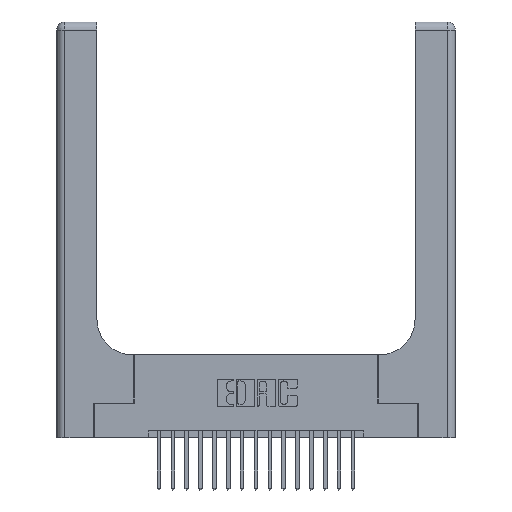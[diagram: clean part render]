
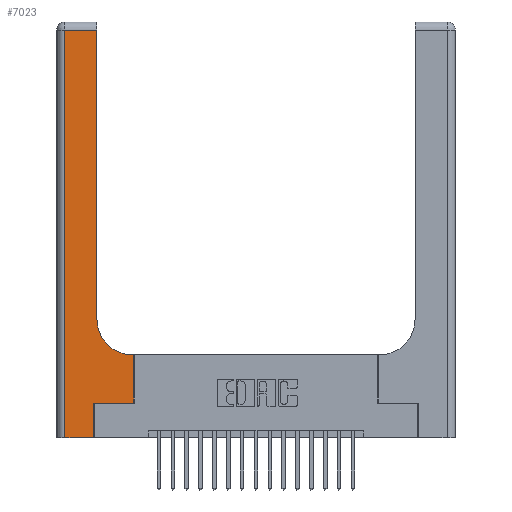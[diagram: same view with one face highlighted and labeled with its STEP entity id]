
A CAD part, top view. The second image highlights one B-rep face of the part: STEP entity #7023.
In plain terms, the highlighted planar face has unit normal (0, 0, 1).
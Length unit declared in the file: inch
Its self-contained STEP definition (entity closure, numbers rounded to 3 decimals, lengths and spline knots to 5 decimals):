
#23 = LINE ( 'NONE', #2422, #16067 ) ;
#148 = VECTOR ( 'NONE', #1297, 39.37008 ) ;
#479 = LINE ( 'NONE', #8664, #4273 ) ;
#485 = DIRECTION ( 'NONE',  ( 1., 0., 0. ) ) ;
#1064 = CARTESIAN_POINT ( 'NONE',  ( 0.06, 2.94, 0.37 ) ) ;
#1297 = DIRECTION ( 'NONE',  ( -1., 0., 0. ) ) ;
#1401 = CARTESIAN_POINT ( 'NONE',  ( 0.2915, 3., 0.37 ) ) ;
#1628 = VERTEX_POINT ( 'NONE', #19528 ) ;
#1999 = LINE ( 'NONE', #17982, #5778 ) ;
#2118 = ORIENTED_EDGE ( 'NONE', *, *, #14097, .T. ) ;
#2130 = CARTESIAN_POINT ( 'NONE',  ( 0.06, 0., 0.37 ) ) ;
#2395 = CARTESIAN_POINT ( 'NONE',  ( 0.5585, 0.25, 0.37 ) ) ;
#2422 = CARTESIAN_POINT ( 'NONE',  ( 0.5585, 0.25, 0.37 ) ) ;
#2802 = ORIENTED_EDGE ( 'NONE', *, *, #19933, .T. ) ;
#3345 = CARTESIAN_POINT ( 'NONE',  ( 0.2915, 0.85, 0.37 ) ) ;
#3592 = EDGE_CURVE ( 'NONE', #9612, #16155, #479, .T. ) ;
#3935 = AXIS2_PLACEMENT_3D ( 'NONE', #5026, #14536, #17753 ) ;
#4273 = VECTOR ( 'NONE', #9222, 39.37008 ) ;
#4458 = LINE ( 'NONE', #6158, #148 ) ;
#5026 = CARTESIAN_POINT ( 'NONE',  ( 0., 3., 0.37 ) ) ;
#5108 = VECTOR ( 'NONE', #8310, 39.37008 ) ;
#5778 = VECTOR ( 'NONE', #6880, 39.37008 ) ;
#5889 = FACE_OUTER_BOUND ( 'NONE', #16660, .T. ) ;
#6094 = LINE ( 'NONE', #17221, #9833 ) ;
#6096 = DIRECTION ( 'NONE',  ( 0., -1., 0. ) ) ;
#6158 = CARTESIAN_POINT ( 'NONE',  ( 0., 2.94, 0.37 ) ) ;
#6204 = CIRCLE ( 'NONE', #20380, 0.25 ) ;
#6464 = VECTOR ( 'NONE', #20124, 39.37008 ) ;
#6644 = PLANE ( 'NONE',  #3935 ) ;
#6880 = DIRECTION ( 'NONE',  ( 0., 1., 0. ) ) ;
#6988 = CARTESIAN_POINT ( 'NONE',  ( 0.269, 0.25, 0.37 ) ) ;
#7023 = ADVANCED_FACE ( 'NONE', ( #5889 ), #6644, .F. ) ;
#7247 = DIRECTION ( 'NONE',  ( 0., 1., 0. ) ) ;
#7655 = CARTESIAN_POINT ( 'NONE',  ( 0.2915, 2.94, 0.37 ) ) ;
#7853 = LINE ( 'NONE', #16240, #5108 ) ;
#8182 = ORIENTED_EDGE ( 'NONE', *, *, #12435, .T. ) ;
#8310 = DIRECTION ( 'NONE',  ( -1., 0., 0. ) ) ;
#8577 = EDGE_CURVE ( 'NONE', #10728, #14247, #18611, .T. ) ;
#8664 = CARTESIAN_POINT ( 'NONE',  ( 0., 0., 0.37 ) ) ;
#8688 = EDGE_CURVE ( 'NONE', #11647, #9305, #4458, .T. ) ;
#9002 = ORIENTED_EDGE ( 'NONE', *, *, #8577, .T. ) ;
#9222 = DIRECTION ( 'NONE',  ( 1., 0., 0. ) ) ;
#9305 = VERTEX_POINT ( 'NONE', #1064 ) ;
#9573 = ORIENTED_EDGE ( 'NONE', *, *, #8688, .T. ) ;
#9612 = VERTEX_POINT ( 'NONE', #2130 ) ;
#9833 = VECTOR ( 'NONE', #6096, 39.37008 ) ;
#10093 = DIRECTION ( 'NONE',  ( 0., 0., -1. ) ) ;
#10425 = ORIENTED_EDGE ( 'NONE', *, *, #17731, .T. ) ;
#10728 = VERTEX_POINT ( 'NONE', #6988 ) ;
#10908 = CARTESIAN_POINT ( 'NONE',  ( 0.5585, 0.6, 0.37 ) ) ;
#10935 = VECTOR ( 'NONE', #14224, 39.37008 ) ;
#10971 = ORIENTED_EDGE ( 'NONE', *, *, #19688, .T. ) ;
#11647 = VERTEX_POINT ( 'NONE', #7655 ) ;
#12234 = ORIENTED_EDGE ( 'NONE', *, *, #3592, .T. ) ;
#12435 = EDGE_CURVE ( 'NONE', #9305, #9612, #6094, .T. ) ;
#14097 = EDGE_CURVE ( 'NONE', #16155, #10728, #1999, .T. ) ;
#14224 = DIRECTION ( 'NONE',  ( 0., 1., 0. ) ) ;
#14247 = VERTEX_POINT ( 'NONE', #2395 ) ;
#14536 = DIRECTION ( 'NONE',  ( 0., 0., -1. ) ) ;
#16067 = VECTOR ( 'NONE', #7247, 39.37008 ) ;
#16155 = VERTEX_POINT ( 'NONE', #20291 ) ;
#16240 = CARTESIAN_POINT ( 'NONE',  ( 0.2915, 0.6, 0.37 ) ) ;
#16660 = EDGE_LOOP ( 'NONE', ( #10425, #9573, #8182, #12234, #2118, #9002, #2802, #10971, #18459 ) ) ;
#16672 = VERTEX_POINT ( 'NONE', #10908 ) ;
#17221 = CARTESIAN_POINT ( 'NONE',  ( 0.06, 3., 0.37 ) ) ;
#17326 = EDGE_CURVE ( 'NONE', #1628, #19629, #6204, .T. ) ;
#17731 = EDGE_CURVE ( 'NONE', #19629, #11647, #19322, .T. ) ;
#17753 = DIRECTION ( 'NONE',  ( -1., 0., 0. ) ) ;
#17982 = CARTESIAN_POINT ( 'NONE',  ( 0.269, 0., 0.37 ) ) ;
#18459 = ORIENTED_EDGE ( 'NONE', *, *, #17326, .T. ) ;
#18563 = CARTESIAN_POINT ( 'NONE',  ( 0.269, 0.25, 0.37 ) ) ;
#18611 = LINE ( 'NONE', #18563, #6464 ) ;
#19322 = LINE ( 'NONE', #1401, #10935 ) ;
#19528 = CARTESIAN_POINT ( 'NONE',  ( 0.5415, 0.6, 0.37 ) ) ;
#19558 = CARTESIAN_POINT ( 'NONE',  ( 0.5415, 0.85, 0.37 ) ) ;
#19629 = VERTEX_POINT ( 'NONE', #3345 ) ;
#19688 = EDGE_CURVE ( 'NONE', #16672, #1628, #7853, .T. ) ;
#19933 = EDGE_CURVE ( 'NONE', #14247, #16672, #23, .T. ) ;
#20124 = DIRECTION ( 'NONE',  ( 1., 0., 0. ) ) ;
#20291 = CARTESIAN_POINT ( 'NONE',  ( 0.269, 0., 0.37 ) ) ;
#20380 = AXIS2_PLACEMENT_3D ( 'NONE', #19558, #10093, #485 ) ;
